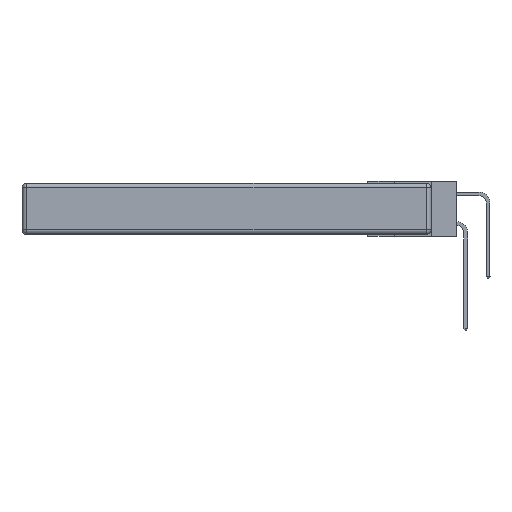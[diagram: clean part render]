
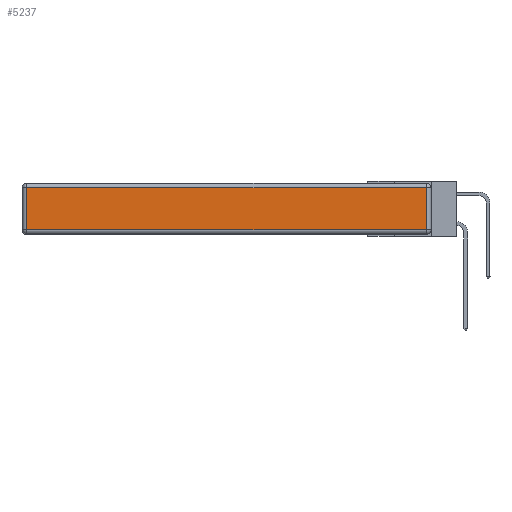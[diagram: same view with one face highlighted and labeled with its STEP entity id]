
A CAD part, left-side view. The second image highlights one B-rep face of the part: STEP entity #5237.
In plain terms, the highlighted planar face has unit normal (-1, 0, 0).
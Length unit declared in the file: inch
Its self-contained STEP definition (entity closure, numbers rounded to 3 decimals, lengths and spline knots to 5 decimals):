
#185 = EDGE_CURVE ( 'NONE', #5102, #5513, #11557, .T. ) ;
#752 = EDGE_CURVE ( 'NONE', #2696, #13004, #7597, .T. ) ;
#814 = CARTESIAN_POINT ( 'NONE',  ( 0., 0.03, -0.343 ) ) ;
#910 = DIRECTION ( 'NONE',  ( 0., 0., 1. ) ) ;
#1134 = EDGE_CURVE ( 'NONE', #5513, #2696, #10996, .T. ) ;
#1769 = CARTESIAN_POINT ( 'NONE',  ( 0., 2.75, -0.03 ) ) ;
#1933 = EDGE_LOOP ( 'NONE', ( #3145, #2280, #12877, #2441 ) ) ;
#1944 = CARTESIAN_POINT ( 'NONE',  ( 0., 0., -0.343 ) ) ;
#2280 = ORIENTED_EDGE ( 'NONE', *, *, #1134, .T. ) ;
#2441 = ORIENTED_EDGE ( 'NONE', *, *, #4147, .T. ) ;
#2515 = CARTESIAN_POINT ( 'NONE',  ( 0., 2.72, -0.03 ) ) ;
#2696 = VERTEX_POINT ( 'NONE', #3755 ) ;
#2875 = CARTESIAN_POINT ( 'NONE',  ( 0., 0.03, -0.313 ) ) ;
#3145 = ORIENTED_EDGE ( 'NONE', *, *, #185, .T. ) ;
#3755 = CARTESIAN_POINT ( 'NONE',  ( 0., 0.03, -0.03 ) ) ;
#3777 = DIRECTION ( 'NONE',  ( 0., 1., 0. ) ) ;
#4147 = EDGE_CURVE ( 'NONE', #13004, #5102, #5024, .T. ) ;
#4823 = CARTESIAN_POINT ( 'NONE',  ( 0., 0., -0.313 ) ) ;
#5024 = LINE ( 'NONE', #8504, #10013 ) ;
#5102 = VERTEX_POINT ( 'NONE', #12669 ) ;
#5237 = ADVANCED_FACE ( 'NONE', ( #13917 ), #8703, .T. ) ;
#5513 = VERTEX_POINT ( 'NONE', #2875 ) ;
#6678 = AXIS2_PLACEMENT_3D ( 'NONE', #1944, #7493, #910 ) ;
#7000 = DIRECTION ( 'NONE',  ( 0., -1., 0. ) ) ;
#7493 = DIRECTION ( 'NONE',  ( -1., 0., 0. ) ) ;
#7597 = LINE ( 'NONE', #1769, #8675 ) ;
#8328 = VECTOR ( 'NONE', #7000, 39.37008 ) ;
#8504 = CARTESIAN_POINT ( 'NONE',  ( 0., 2.72, -0.343 ) ) ;
#8675 = VECTOR ( 'NONE', #3777, 39.37008 ) ;
#8703 = PLANE ( 'NONE',  #6678 ) ;
#10013 = VECTOR ( 'NONE', #11911, 39.37008 ) ;
#10996 = LINE ( 'NONE', #814, #11345 ) ;
#11345 = VECTOR ( 'NONE', #13129, 39.37008 ) ;
#11557 = LINE ( 'NONE', #4823, #8328 ) ;
#11911 = DIRECTION ( 'NONE',  ( 0., 0., -1. ) ) ;
#12669 = CARTESIAN_POINT ( 'NONE',  ( 0., 2.72, -0.313 ) ) ;
#12877 = ORIENTED_EDGE ( 'NONE', *, *, #752, .T. ) ;
#13004 = VERTEX_POINT ( 'NONE', #2515 ) ;
#13129 = DIRECTION ( 'NONE',  ( 0., 0., 1. ) ) ;
#13917 = FACE_OUTER_BOUND ( 'NONE', #1933, .T. ) ;
